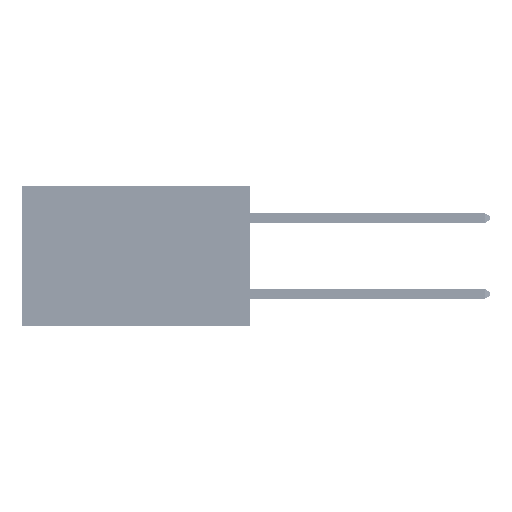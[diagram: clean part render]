
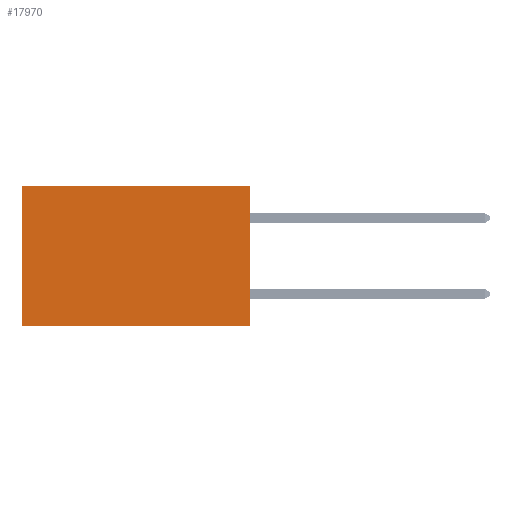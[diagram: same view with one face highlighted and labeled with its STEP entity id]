
A CAD part, left-side view. The second image highlights one B-rep face of the part: STEP entity #17970.
In plain terms, the highlighted planar face has unit normal (-1, 0, 0).
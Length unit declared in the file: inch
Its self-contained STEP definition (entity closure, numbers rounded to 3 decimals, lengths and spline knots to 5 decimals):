
#174 = PLANE ( 'NONE',  #40704 ) ;
#3738 = LINE ( 'NONE', #27843, #27960 ) ;
#4299 = LINE ( 'NONE', #28354, #13159 ) ;
#5855 = FACE_OUTER_BOUND ( 'NONE', #17651, .T. ) ;
#5858 = ORIENTED_EDGE ( 'NONE', *, *, #39293, .T. ) ;
#8333 = CARTESIAN_POINT ( 'NONE',  ( 0.2875, 0., 0. ) ) ;
#8962 = CARTESIAN_POINT ( 'NONE',  ( 0.2875, 0.6, 0. ) ) ;
#10310 = VERTEX_POINT ( 'NONE', #8962 ) ;
#11369 = DIRECTION ( 'NONE',  ( 0., 0., -1. ) ) ;
#13159 = VECTOR ( 'NONE', #13313, 39.37008 ) ;
#13162 = CARTESIAN_POINT ( 'NONE',  ( 0.2875, 0., -0.37 ) ) ;
#13313 = DIRECTION ( 'NONE',  ( 0., 1., 0. ) ) ;
#15725 = EDGE_CURVE ( 'NONE', #24230, #10310, #4299, .T. ) ;
#17651 = EDGE_LOOP ( 'NONE', ( #5858, #40895, #43078, #22409 ) ) ;
#17970 = ADVANCED_FACE ( 'NONE', ( #5855 ), #174, .F. ) ;
#18206 = VECTOR ( 'NONE', #30833, 39.37008 ) ;
#18767 = LINE ( 'NONE', #8333, #18206 ) ;
#20112 = EDGE_CURVE ( 'NONE', #30169, #41210, #3738, .T. ) ;
#20246 = DIRECTION ( 'NONE',  ( 0., 1., 0. ) ) ;
#22409 = ORIENTED_EDGE ( 'NONE', *, *, #15725, .T. ) ;
#22758 = VECTOR ( 'NONE', #11369, 39.37008 ) ;
#23751 = EDGE_CURVE ( 'NONE', #24230, #30169, #18767, .T. ) ;
#23937 = CARTESIAN_POINT ( 'NONE',  ( 0.2875, 0.6, -0.37 ) ) ;
#24230 = VERTEX_POINT ( 'NONE', #45699 ) ;
#27843 = CARTESIAN_POINT ( 'NONE',  ( 0.2875, 0., -0.37 ) ) ;
#27960 = VECTOR ( 'NONE', #20246, 39.37008 ) ;
#28354 = CARTESIAN_POINT ( 'NONE',  ( 0.2875, 0., 0. ) ) ;
#30169 = VERTEX_POINT ( 'NONE', #13162 ) ;
#30426 = DIRECTION ( 'NONE',  ( 1., 0., 0. ) ) ;
#30833 = DIRECTION ( 'NONE',  ( 0., 0., -1. ) ) ;
#34757 = CARTESIAN_POINT ( 'NONE',  ( 0.2875, 0., 0. ) ) ;
#37217 = CARTESIAN_POINT ( 'NONE',  ( 0.2875, 0.6, 0. ) ) ;
#39293 = EDGE_CURVE ( 'NONE', #10310, #41210, #48811, .T. ) ;
#40704 = AXIS2_PLACEMENT_3D ( 'NONE', #34757, #30426, #46146 ) ;
#40895 = ORIENTED_EDGE ( 'NONE', *, *, #20112, .F. ) ;
#41210 = VERTEX_POINT ( 'NONE', #23937 ) ;
#43078 = ORIENTED_EDGE ( 'NONE', *, *, #23751, .F. ) ;
#45699 = CARTESIAN_POINT ( 'NONE',  ( 0.2875, 0., 0. ) ) ;
#46146 = DIRECTION ( 'NONE',  ( 0., 0., -1. ) ) ;
#48811 = LINE ( 'NONE', #37217, #22758 ) ;
